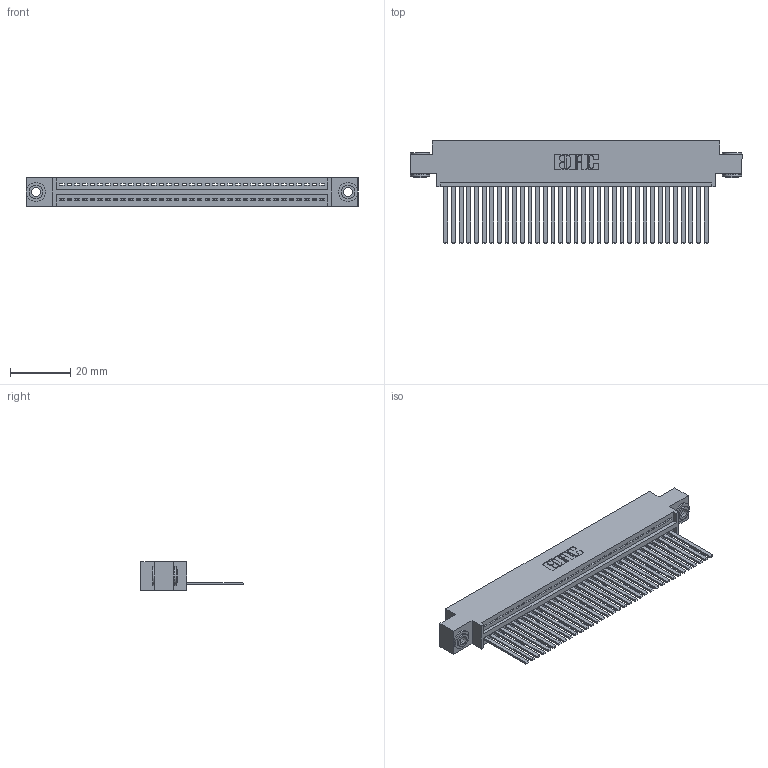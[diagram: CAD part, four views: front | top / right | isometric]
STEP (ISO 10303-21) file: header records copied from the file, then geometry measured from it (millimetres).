
FILE_DESCRIPTION (( 'STEP AP203' ), '1' );
FILE_NAME ('345-035-544-603.STEP', '2018-08-29T07:38:16', ( '' ), ( '' ), 'SwSTEP 2.0', 'SolidWorks 2016', '' );
FILE_SCHEMA (( 'CONFIG_CONTROL_DESIGN' ));
Length unit declared in the file: inch
Products named in the file (4): 345-250-002_345-250-002-102; 345-035-544-603; 345 Part_0.170 Offset - 0.156 Dia-TH; 345-292-001_345-293-144
Assembly tree (38 placements, depth 2):
  345-035-544-603
    345 Part_0.170 Offset - 0.156 Dia-TH
    345-292-001_345-293-144  x35
    345-250-002_345-250-002-102  x2
Bounding box: 110.11 x 33.96 x 9.4 mm (x, y, z)
Volume: 10712.3 mm3; surface area: 15698.4 mm2
Topology: 38 solids, 38 shells, 1988 faces, 5959 edges, 3922 vertices
Faces by surface type: plane 1354, cylinder 626, cone 8
Entity records: 27882 total; most frequent: CARTESIAN_POINT 4808, ORIENTED_EDGE 4770, DIRECTION 4237, EDGE_CURVE 2385, VECTOR 2093, LINE 2093, VERTEX_POINT 1586, AXIS2_PLACEMENT_3D 1072
